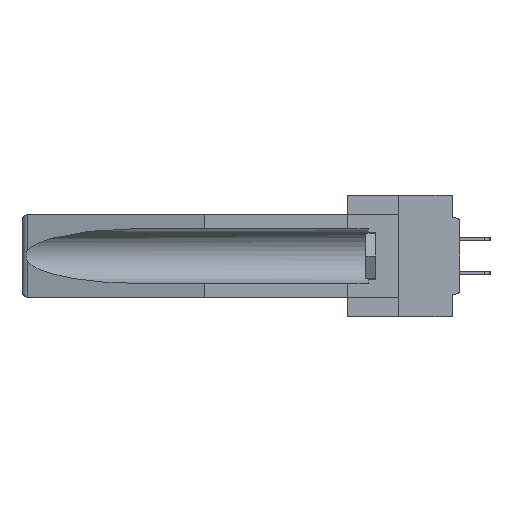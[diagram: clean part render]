
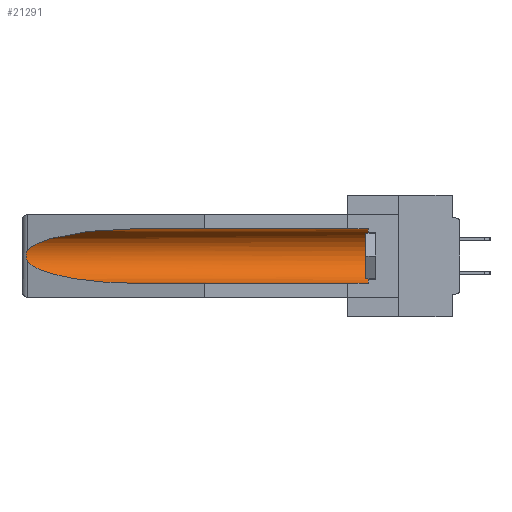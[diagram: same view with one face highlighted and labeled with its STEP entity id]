
A CAD part, left-side view. The second image highlights one B-rep face of the part: STEP entity #21291.
In plain terms, the highlighted cylindrical face has radius 2.857 mm (diameter 5.715 mm), a partial arc.
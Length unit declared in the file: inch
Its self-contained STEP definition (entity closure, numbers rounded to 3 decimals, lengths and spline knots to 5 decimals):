
#102 = EDGE_CURVE ( 'NONE', #16638, #12526, #24118, .T. ) ;
#727 = VERTEX_POINT ( 'NONE', #21856 ) ;
#918 = CYLINDRICAL_SURFACE ( 'NONE', #27323, 0.1125 ) ;
#1330 = ORIENTED_EDGE ( 'NONE', *, *, #18503, .T. ) ;
#2885 = ORIENTED_EDGE ( 'NONE', *, *, #7416, .T. ) ;
#3598 = VERTEX_POINT ( 'NONE', #12861 ) ;
#6839 = CIRCLE ( 'NONE', #38863, 0.1125 ) ;
#7416 = EDGE_CURVE ( 'NONE', #3598, #10183, #16175, .T. ) ;
#7514 = CARTESIAN_POINT ( 'NONE',  ( 0.21114, 1.30732, -0.059 ) ) ;
#7812 = VECTOR ( 'NONE', #28766, 39.37008 ) ;
#8382 = VERTEX_POINT ( 'NONE', #29313 ) ;
#10183 = VERTEX_POINT ( 'NONE', #26720 ) ;
#10372 = DIRECTION ( 'NONE',  ( 0., 1., 0. ) ) ;
#10509 = CARTESIAN_POINT ( 'NONE',  ( 0.2675, 1.53308, -0.16763 ) ) ;
#10763 = CARTESIAN_POINT ( 'NONE',  ( 0.2675, 1.53308, -0.17534 ) ) ;
#12526 = VERTEX_POINT ( 'NONE', #16329 ) ;
#12861 = CARTESIAN_POINT ( 'NONE',  ( 0.155, 1.07973, -0.059 ) ) ;
#13155 = CARTESIAN_POINT ( 'NONE',  ( 0.155, 1.07973, -0.284 ) ) ;
#13553 = CARTESIAN_POINT ( 'NONE',  ( 0.2673, 1.53269, -0.17917 ) ) ;
#14728 = DIRECTION ( 'NONE',  ( 0., 0., 1. ) ) ;
#16175 =( BOUNDED_CURVE ( )  B_SPLINE_CURVE ( 3, ( #31957, #7514, #23098, #29054 ),
 .UNSPECIFIED., .F., .F. ) 
 B_SPLINE_CURVE_WITH_KNOTS ( ( 4, 4 ),
 ( 4.71239, 6.08839 ),
 .UNSPECIFIED. ) 
 CURVE ( )  GEOMETRIC_REPRESENTATION_ITEM ( )  RATIONAL_B_SPLINE_CURVE ( ( 1., 0.848, 0.848, 1. ) ) 
 REPRESENTATION_ITEM ( '' )  );
#16329 = CARTESIAN_POINT ( 'NONE',  ( 0.155, 1.07973, -0.284 ) ) ;
#16343 = CARTESIAN_POINT ( 'NONE',  ( 0.26537, 1.52718, -0.14972 ) ) ;
#16348 = EDGE_CURVE ( 'NONE', #8382, #12526, #26795, .T. ) ;
#16638 = VERTEX_POINT ( 'NONE', #17510 ) ;
#17510 = CARTESIAN_POINT ( 'NONE',  ( 0.155, 0.126, -0.284 ) ) ;
#17645 = DIRECTION ( 'NONE',  ( 0., -1., 0. ) ) ;
#17732 = EDGE_LOOP ( 'NONE', ( #2885, #29858, #23530, #32989, #33148, #1330 ) ) ;
#18503 = EDGE_CURVE ( 'NONE', #727, #3598, #31479, .T. ) ;
#18683 = EDGE_CURVE ( 'NONE', #16638, #727, #6839, .T. ) ;
#19541 = CARTESIAN_POINT ( 'NONE',  ( 0.26654, 1.53092, -0.15636 ) ) ;
#21291 = ADVANCED_FACE ( 'NONE', ( #31708 ), #918, .F. ) ;
#21856 = CARTESIAN_POINT ( 'NONE',  ( 0.155, 0.126, -0.059 ) ) ;
#22294 = CARTESIAN_POINT ( 'NONE',  ( 0.25451, 1.48313, -0.24835 ) ) ;
#23098 = CARTESIAN_POINT ( 'NONE',  ( 0.25451, 1.48313, -0.09465 ) ) ;
#23530 = ORIENTED_EDGE ( 'NONE', *, *, #16348, .T. ) ;
#24118 = LINE ( 'NONE', #31544, #25529 ) ;
#25069 = CARTESIAN_POINT ( 'NONE',  ( 0.26537, 1.52718, -0.19328 ) ) ;
#25529 = VECTOR ( 'NONE', #10372, 39.37008 ) ;
#25603 = CARTESIAN_POINT ( 'NONE',  ( 0.155, -0.30754, -0.059 ) ) ;
#26720 = CARTESIAN_POINT ( 'NONE',  ( 0.26537, 1.52718, -0.14972 ) ) ;
#26795 =( BOUNDED_CURVE ( )  B_SPLINE_CURVE ( 3, ( #25069, #22294, #28243, #13155 ),
 .UNSPECIFIED., .F., .F. ) 
 B_SPLINE_CURVE_WITH_KNOTS ( ( 4, 4 ),
 ( 0.1948, 1.5708 ),
 .UNSPECIFIED. ) 
 CURVE ( )  GEOMETRIC_REPRESENTATION_ITEM ( )  RATIONAL_B_SPLINE_CURVE ( ( 1., 0.848, 0.848, 1. ) ) 
 REPRESENTATION_ITEM ( '' )  );
#27013 = CARTESIAN_POINT ( 'NONE',  ( 0.155, 0.126, -0.1715 ) ) ;
#27323 = AXIS2_PLACEMENT_3D ( 'NONE', #28104, #37054, #28232 ) ;
#28104 = CARTESIAN_POINT ( 'NONE',  ( 0.155, -0.30754, -0.1715 ) ) ;
#28232 = DIRECTION ( 'NONE',  ( 0., 0., 1. ) ) ;
#28243 = CARTESIAN_POINT ( 'NONE',  ( 0.21114, 1.30732, -0.284 ) ) ;
#28637 = CARTESIAN_POINT ( 'NONE',  ( 0.2673, 1.5327, -0.16383 ) ) ;
#28766 = DIRECTION ( 'NONE',  ( 0., 1., 0. ) ) ;
#29054 = CARTESIAN_POINT ( 'NONE',  ( 0.26537, 1.52718, -0.14972 ) ) ;
#29313 = CARTESIAN_POINT ( 'NONE',  ( 0.26537, 1.52718, -0.19328 ) ) ;
#29858 = ORIENTED_EDGE ( 'NONE', *, *, #37547, .T. ) ;
#31479 = LINE ( 'NONE', #25603, #7812 ) ;
#31544 = CARTESIAN_POINT ( 'NONE',  ( 0.155, -0.30754, -0.284 ) ) ;
#31708 = FACE_OUTER_BOUND ( 'NONE', #17732, .T. ) ;
#31957 = CARTESIAN_POINT ( 'NONE',  ( 0.155, 1.07973, -0.059 ) ) ;
#32137 = B_SPLINE_CURVE_WITH_KNOTS ( 'NONE', 3,
 ( #16343, #37581, #19541, #28637, #10509, #10763, #13553, #34674, #34937, #38361 ),
 .UNSPECIFIED., .F., .F.,
 ( 4, 2, 2, 2, 4 ),
 ( 0., 0.00029, 0.00058, 0.00087, 0.00117 ),
 .UNSPECIFIED. ) ;
#32989 = ORIENTED_EDGE ( 'NONE', *, *, #102, .F. ) ;
#33148 = ORIENTED_EDGE ( 'NONE', *, *, #18683, .T. ) ;
#34674 = CARTESIAN_POINT ( 'NONE',  ( 0.26655, 1.53094, -0.18657 ) ) ;
#34937 = CARTESIAN_POINT ( 'NONE',  ( 0.26597, 1.5296, -0.19026 ) ) ;
#37054 = DIRECTION ( 'NONE',  ( 0., 1., 0. ) ) ;
#37547 = EDGE_CURVE ( 'NONE', #10183, #8382, #32137, .T. ) ;
#37581 = CARTESIAN_POINT ( 'NONE',  ( 0.26597, 1.52961, -0.15275 ) ) ;
#38361 = CARTESIAN_POINT ( 'NONE',  ( 0.26537, 1.52718, -0.19328 ) ) ;
#38863 = AXIS2_PLACEMENT_3D ( 'NONE', #27013, #17645, #14728 ) ;
